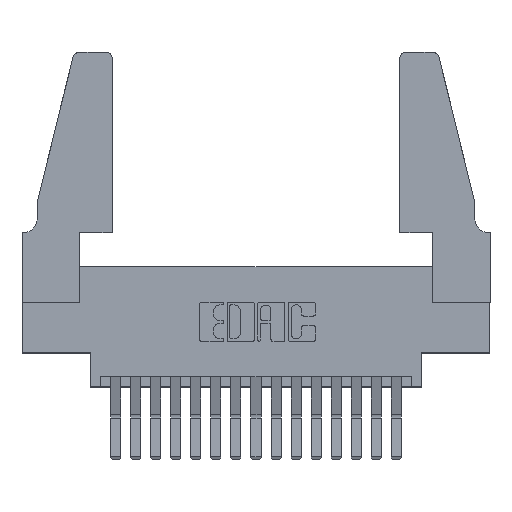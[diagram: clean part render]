
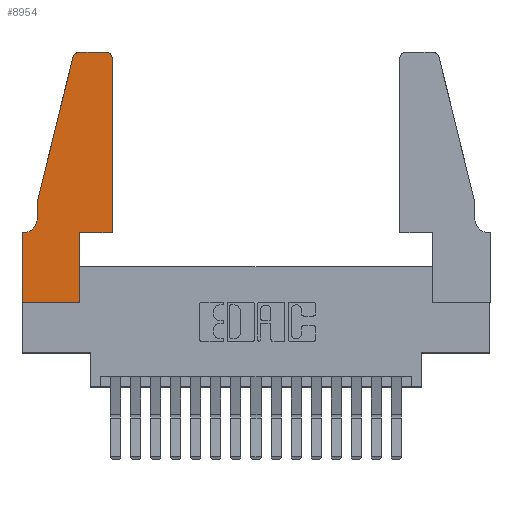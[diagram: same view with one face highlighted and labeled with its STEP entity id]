
A CAD part, top view. The second image highlights one B-rep face of the part: STEP entity #8954.
In plain terms, the highlighted planar face has unit normal (0, 0, 1).
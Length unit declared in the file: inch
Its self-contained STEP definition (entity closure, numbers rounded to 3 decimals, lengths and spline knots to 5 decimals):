
#29 = ORIENTED_EDGE ( 'NONE', *, *, #6322, .T. ) ;
#250 = VERTEX_POINT ( 'NONE', #1027 ) ;
#378 = ORIENTED_EDGE ( 'NONE', *, *, #14411, .T. ) ;
#595 = ORIENTED_EDGE ( 'NONE', *, *, #14251, .T. ) ;
#896 = CARTESIAN_POINT ( 'NONE',  ( 0.4505, 0.35, 0.37 ) ) ;
#1027 = CARTESIAN_POINT ( 'NONE',  ( 0.4505, 0.35, 0.37 ) ) ;
#1066 = AXIS2_PLACEMENT_3D ( 'NONE', #13836, #16593, #8393 ) ;
#1186 = EDGE_CURVE ( 'NONE', #9210, #13714, #11166, .T. ) ;
#1282 = EDGE_CURVE ( 'NONE', #14894, #9878, #4498, .T. ) ;
#1946 = AXIS2_PLACEMENT_3D ( 'NONE', #6777, #4256, #8292 ) ;
#1977 = DIRECTION ( 'NONE',  ( -1., 0., 0. ) ) ;
#2073 = LINE ( 'NONE', #12969, #8357 ) ;
#2382 = CARTESIAN_POINT ( 'NONE',  ( 0.0755, 0.5, 0.37 ) ) ;
#2438 = DIRECTION ( 'NONE',  ( -1., 0., 0. ) ) ;
#2718 = DIRECTION ( 'NONE',  ( 1., 0., 0. ) ) ;
#2875 = FACE_OUTER_BOUND ( 'NONE', #6300, .T. ) ;
#3009 = DIRECTION ( 'NONE',  ( 0., 1., 0. ) ) ;
#3276 = ORIENTED_EDGE ( 'NONE', *, *, #1282, .T. ) ;
#3306 = CIRCLE ( 'NONE', #17058, 0.03 ) ;
#3856 = VECTOR ( 'NONE', #4873, 39.37008 ) ;
#4025 = DIRECTION ( 'NONE',  ( 1., 0., 0. ) ) ;
#4256 = DIRECTION ( 'NONE',  ( 0., 0., 1. ) ) ;
#4498 = CIRCLE ( 'NONE', #1066, 0.03 ) ;
#4581 = CARTESIAN_POINT ( 'NONE',  ( 0.4205, 1.25, 0.37 ) ) ;
#4873 = DIRECTION ( 'NONE',  ( 0., 1., 0. ) ) ;
#5283 = EDGE_CURVE ( 'NONE', #250, #14894, #13298, .T. ) ;
#5449 = DIRECTION ( 'NONE',  ( 0., 0., -1. ) ) ;
#6002 = CARTESIAN_POINT ( 'NONE',  ( 0.0755, 0.35, 0.37 ) ) ;
#6300 = EDGE_LOOP ( 'NONE', ( #29, #8361, #378, #6972, #12776, #15184, #16907, #16934, #7047, #595, #17022, #3276 ) ) ;
#6322 = EDGE_CURVE ( 'NONE', #9878, #12909, #2073, .T. ) ;
#6527 = DIRECTION ( 'NONE',  ( -0.239, -0.971, 0. ) ) ;
#6777 = CARTESIAN_POINT ( 'NONE',  ( 0., 0.35, 0.37 ) ) ;
#6972 = ORIENTED_EDGE ( 'NONE', *, *, #16023, .T. ) ;
#7047 = ORIENTED_EDGE ( 'NONE', *, *, #13018, .T. ) ;
#7384 = DIRECTION ( 'NONE',  ( -1., 0., 0. ) ) ;
#7537 = CARTESIAN_POINT ( 'NONE',  ( 0.4505, 1.22, 0.37 ) ) ;
#7558 = CIRCLE ( 'NONE', #15831, 0.07 ) ;
#8270 = EDGE_CURVE ( 'NONE', #16889, #11977, #14477, .T. ) ;
#8292 = DIRECTION ( 'NONE',  ( 1., 0., 0. ) ) ;
#8307 = VECTOR ( 'NONE', #7384, 39.37008 ) ;
#8344 = DIRECTION ( 'NONE',  ( 1., 0., 0. ) ) ;
#8357 = VECTOR ( 'NONE', #1977, 39.37008 ) ;
#8361 = ORIENTED_EDGE ( 'NONE', *, *, #10692, .T. ) ;
#8393 = DIRECTION ( 'NONE',  ( 1., 0., 0. ) ) ;
#8807 = CARTESIAN_POINT ( 'NONE',  ( 0.2865, 0.35, 0.37 ) ) ;
#8954 = ADVANCED_FACE ( 'NONE', ( #2875 ), #13603, .T. ) ;
#9210 = VERTEX_POINT ( 'NONE', #9686 ) ;
#9686 = CARTESIAN_POINT ( 'NONE',  ( 0., 0., 0.37 ) ) ;
#9878 = VERTEX_POINT ( 'NONE', #4581 ) ;
#10200 = CARTESIAN_POINT ( 'NONE',  ( 0.2865, 0., 0.37 ) ) ;
#10415 = CARTESIAN_POINT ( 'NONE',  ( 0., 0.35, 0.37 ) ) ;
#10641 = VERTEX_POINT ( 'NONE', #12226 ) ;
#10644 = VECTOR ( 'NONE', #15795, 39.37008 ) ;
#10692 = EDGE_CURVE ( 'NONE', #12909, #10641, #3306, .T. ) ;
#11166 = LINE ( 'NONE', #15099, #16090 ) ;
#11270 = CARTESIAN_POINT ( 'NONE',  ( 0., 0., 0.37 ) ) ;
#11589 = VERTEX_POINT ( 'NONE', #17272 ) ;
#11977 = VERTEX_POINT ( 'NONE', #10415 ) ;
#12226 = CARTESIAN_POINT ( 'NONE',  ( 0.25487, 1.22718, 0.37 ) ) ;
#12776 = ORIENTED_EDGE ( 'NONE', *, *, #16658, .T. ) ;
#12810 = CARTESIAN_POINT ( 'NONE',  ( 0.284, 1.25, 0.37 ) ) ;
#12909 = VERTEX_POINT ( 'NONE', #12810 ) ;
#12969 = CARTESIAN_POINT ( 'NONE',  ( 0.2605, 1.25, 0.37 ) ) ;
#13018 = EDGE_CURVE ( 'NONE', #13714, #14676, #17798, .T. ) ;
#13022 = LINE ( 'NONE', #896, #14094 ) ;
#13239 = LINE ( 'NONE', #14488, #13896 ) ;
#13298 = LINE ( 'NONE', #14701, #3856 ) ;
#13583 = EDGE_CURVE ( 'NONE', #11977, #9210, #13915, .T. ) ;
#13603 = PLANE ( 'NONE',  #1946 ) ;
#13670 = CARTESIAN_POINT ( 'NONE',  ( 0.0055, 0.42, 0.37 ) ) ;
#13714 = VERTEX_POINT ( 'NONE', #10200 ) ;
#13836 = CARTESIAN_POINT ( 'NONE',  ( 0.4205, 1.22, 0.37 ) ) ;
#13843 = LINE ( 'NONE', #17197, #10644 ) ;
#13896 = VECTOR ( 'NONE', #6527, 39.37008 ) ;
#13915 = LINE ( 'NONE', #11270, #15211 ) ;
#14094 = VECTOR ( 'NONE', #4025, 39.37008 ) ;
#14251 = EDGE_CURVE ( 'NONE', #14676, #250, #13022, .T. ) ;
#14411 = EDGE_CURVE ( 'NONE', #10641, #16002, #13239, .T. ) ;
#14477 = LINE ( 'NONE', #6002, #8307 ) ;
#14488 = CARTESIAN_POINT ( 'NONE',  ( 0.0755, 0.5, 0.37 ) ) ;
#14676 = VERTEX_POINT ( 'NONE', #8807 ) ;
#14701 = CARTESIAN_POINT ( 'NONE',  ( 0.4505, 0.35, 0.37 ) ) ;
#14894 = VERTEX_POINT ( 'NONE', #7537 ) ;
#14956 = CARTESIAN_POINT ( 'NONE',  ( 0.284, 1.22, 0.37 ) ) ;
#15080 = DIRECTION ( 'NONE',  ( 0., 0., 1. ) ) ;
#15084 = CARTESIAN_POINT ( 'NONE',  ( 0.0055, 0.35, 0.37 ) ) ;
#15099 = CARTESIAN_POINT ( 'NONE',  ( 0., 0., 0.37 ) ) ;
#15166 = DIRECTION ( 'NONE',  ( 0., -1., 0. ) ) ;
#15184 = ORIENTED_EDGE ( 'NONE', *, *, #8270, .T. ) ;
#15211 = VECTOR ( 'NONE', #15166, 39.37008 ) ;
#15238 = VECTOR ( 'NONE', #3009, 39.37008 ) ;
#15795 = DIRECTION ( 'NONE',  ( 0., -1., 0. ) ) ;
#15831 = AXIS2_PLACEMENT_3D ( 'NONE', #13670, #5449, #2438 ) ;
#16002 = VERTEX_POINT ( 'NONE', #2382 ) ;
#16023 = EDGE_CURVE ( 'NONE', #16002, #11589, #13843, .T. ) ;
#16090 = VECTOR ( 'NONE', #8344, 39.37008 ) ;
#16593 = DIRECTION ( 'NONE',  ( 0., 0., 1. ) ) ;
#16621 = CARTESIAN_POINT ( 'NONE',  ( 0.2865, 0.35, 0.37 ) ) ;
#16658 = EDGE_CURVE ( 'NONE', #11589, #16889, #7558, .T. ) ;
#16889 = VERTEX_POINT ( 'NONE', #15084 ) ;
#16907 = ORIENTED_EDGE ( 'NONE', *, *, #13583, .T. ) ;
#16934 = ORIENTED_EDGE ( 'NONE', *, *, #1186, .T. ) ;
#17022 = ORIENTED_EDGE ( 'NONE', *, *, #5283, .T. ) ;
#17058 = AXIS2_PLACEMENT_3D ( 'NONE', #14956, #15080, #2718 ) ;
#17197 = CARTESIAN_POINT ( 'NONE',  ( 0.0755, 0.5, 0.37 ) ) ;
#17272 = CARTESIAN_POINT ( 'NONE',  ( 0.0755, 0.42, 0.37 ) ) ;
#17798 = LINE ( 'NONE', #16621, #15238 ) ;
